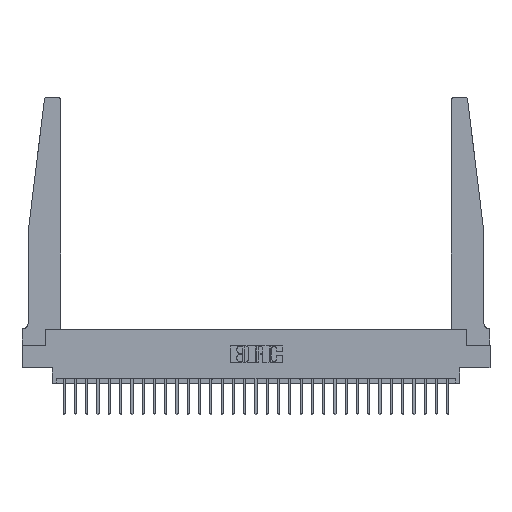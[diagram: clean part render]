
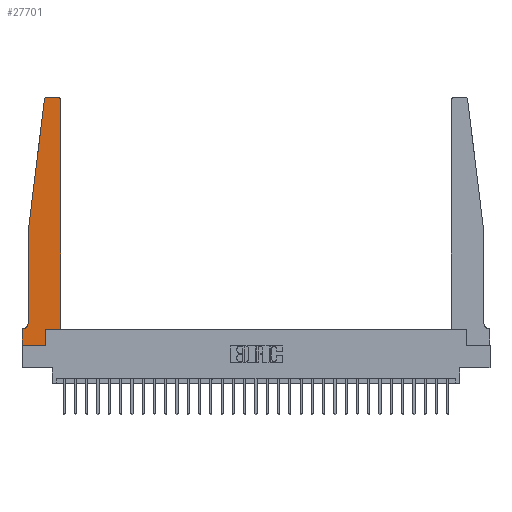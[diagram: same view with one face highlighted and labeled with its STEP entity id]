
A CAD part, top view. The second image highlights one B-rep face of the part: STEP entity #27701.
In plain terms, the highlighted planar face has unit normal (0, 0, 1).
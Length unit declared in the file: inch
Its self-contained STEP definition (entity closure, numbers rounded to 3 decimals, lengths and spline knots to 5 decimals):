
#73 = DIRECTION ( 'NONE',  ( 1., 0., 0. ) ) ;
#163 = EDGE_CURVE ( 'NONE', #21040, #22518, #10459, .T. ) ;
#365 = CARTESIAN_POINT ( 'NONE',  ( 0., 0.1875, 0.37 ) ) ;
#711 = AXIS2_PLACEMENT_3D ( 'NONE', #4234, #19863, #17510 ) ;
#862 = CARTESIAN_POINT ( 'NONE',  ( 0.065, 0.1875, 0.37 ) ) ;
#881 = ORIENTED_EDGE ( 'NONE', *, *, #22320, .T. ) ;
#935 = AXIS2_PLACEMENT_3D ( 'NONE', #18233, #27815, #20877 ) ;
#1850 = CARTESIAN_POINT ( 'NONE',  ( 0.065, 1.25, 0.37 ) ) ;
#1932 = VERTEX_POINT ( 'NONE', #9917 ) ;
#2770 = DIRECTION ( 'NONE',  ( -1., 0., 0. ) ) ;
#3174 = LINE ( 'NONE', #5829, #12867 ) ;
#3251 = VERTEX_POINT ( 'NONE', #11386 ) ;
#3259 = VERTEX_POINT ( 'NONE', #11244 ) ;
#3402 = VERTEX_POINT ( 'NONE', #12240 ) ;
#3509 = DIRECTION ( 'NONE',  ( -0.122, -0.992, 0. ) ) ;
#3838 = VECTOR ( 'NONE', #12747, 39.37008 ) ;
#4233 = CARTESIAN_POINT ( 'NONE',  ( 0.2605, 0., 0.37 ) ) ;
#4234 = CARTESIAN_POINT ( 'NONE',  ( 0.015, 0.2375, 0.37 ) ) ;
#4310 = AXIS2_PLACEMENT_3D ( 'NONE', #365, #22187, #73 ) ;
#5100 = EDGE_LOOP ( 'NONE', ( #24812, #6718, #881, #24952, #23023, #23463, #5910, #11214, #28341, #9028, #5657, #17449 ) ) ;
#5166 = DIRECTION ( 'NONE',  ( -1., 0., 0. ) ) ;
#5617 = EDGE_CURVE ( 'NONE', #22518, #3259, #21421, .T. ) ;
#5657 = ORIENTED_EDGE ( 'NONE', *, *, #10068, .T. ) ;
#5829 = CARTESIAN_POINT ( 'NONE',  ( 0.2605, 0.18, 0.37 ) ) ;
#5910 = ORIENTED_EDGE ( 'NONE', *, *, #23990, .T. ) ;
#5997 = EDGE_CURVE ( 'NONE', #26243, #26681, #3174, .T. ) ;
#6176 = CARTESIAN_POINT ( 'NONE',  ( 0.065, 0.2375, 0.37 ) ) ;
#6427 = DIRECTION ( 'NONE',  ( 1., 0., 0. ) ) ;
#6718 = ORIENTED_EDGE ( 'NONE', *, *, #10291, .T. ) ;
#6726 = VERTEX_POINT ( 'NONE', #6966 ) ;
#6865 = AXIS2_PLACEMENT_3D ( 'NONE', #16122, #15843, #8772 ) ;
#6966 = CARTESIAN_POINT ( 'NONE',  ( 0.395, 2.75, 0.37 ) ) ;
#7486 = EDGE_CURVE ( 'NONE', #3251, #26243, #28417, .T. ) ;
#8772 = DIRECTION ( 'NONE',  ( 1., 0., 0. ) ) ;
#9028 = ORIENTED_EDGE ( 'NONE', *, *, #27541, .T. ) ;
#9371 = VECTOR ( 'NONE', #17293, 39.37008 ) ;
#9666 = VECTOR ( 'NONE', #2770, 39.37008 ) ;
#9760 = VERTEX_POINT ( 'NONE', #28784 ) ;
#9917 = CARTESIAN_POINT ( 'NONE',  ( 0.27653, 2.75, 0.37 ) ) ;
#10068 = EDGE_CURVE ( 'NONE', #10668, #9760, #12353, .T. ) ;
#10291 = EDGE_CURVE ( 'NONE', #1932, #3402, #17422, .T. ) ;
#10459 = LINE ( 'NONE', #28171, #25637 ) ;
#10668 = VERTEX_POINT ( 'NONE', #22879 ) ;
#11214 = ORIENTED_EDGE ( 'NONE', *, *, #7486, .T. ) ;
#11244 = CARTESIAN_POINT ( 'NONE',  ( 0.015, 0.1875, 0.37 ) ) ;
#11386 = CARTESIAN_POINT ( 'NONE',  ( 0., 0., 0.37 ) ) ;
#11794 = CARTESIAN_POINT ( 'NONE',  ( 0.25, 2.75, 0.37 ) ) ;
#12169 = DIRECTION ( 'NONE',  ( 0., 1., 0. ) ) ;
#12218 = LINE ( 'NONE', #14584, #18756 ) ;
#12240 = CARTESIAN_POINT ( 'NONE',  ( 0.24675, 2.72367, 0.37 ) ) ;
#12353 = LINE ( 'NONE', #25790, #18884 ) ;
#12489 = CIRCLE ( 'NONE', #6865, 0.03 ) ;
#12747 = DIRECTION ( 'NONE',  ( 1., 0., 0. ) ) ;
#12867 = VECTOR ( 'NONE', #12169, 39.37008 ) ;
#14584 = CARTESIAN_POINT ( 'NONE',  ( 0.065, 1.25, 0.37 ) ) ;
#15843 = DIRECTION ( 'NONE',  ( 0., 0., 1. ) ) ;
#16122 = CARTESIAN_POINT ( 'NONE',  ( 0.395, 2.72, 0.37 ) ) ;
#16228 = LINE ( 'NONE', #11794, #22544 ) ;
#16712 = LINE ( 'NONE', #23620, #9371 ) ;
#17106 = EDGE_CURVE ( 'NONE', #9760, #6726, #12489, .T. ) ;
#17293 = DIRECTION ( 'NONE',  ( 0., -1., 0. ) ) ;
#17422 = CIRCLE ( 'NONE', #935, 0.03 ) ;
#17449 = ORIENTED_EDGE ( 'NONE', *, *, #17106, .T. ) ;
#17510 = DIRECTION ( 'NONE',  ( -1., 0., 0. ) ) ;
#17772 = CARTESIAN_POINT ( 'NONE',  ( 0., 0., 0.37 ) ) ;
#18233 = CARTESIAN_POINT ( 'NONE',  ( 0.27653, 2.72, 0.37 ) ) ;
#18700 = LINE ( 'NONE', #862, #9666 ) ;
#18756 = VECTOR ( 'NONE', #3509, 39.37008 ) ;
#18884 = VECTOR ( 'NONE', #19576, 39.37008 ) ;
#18886 = EDGE_CURVE ( 'NONE', #3259, #24795, #18700, .T. ) ;
#19576 = DIRECTION ( 'NONE',  ( 0., 1., 0. ) ) ;
#19863 = DIRECTION ( 'NONE',  ( 0., 0., -1. ) ) ;
#19985 = PLANE ( 'NONE',  #4310 ) ;
#20385 = VECTOR ( 'NONE', #6427, 39.37008 ) ;
#20877 = DIRECTION ( 'NONE',  ( 1., 0., 0. ) ) ;
#21040 = VERTEX_POINT ( 'NONE', #1850 ) ;
#21370 = DIRECTION ( 'NONE',  ( 0., -1., 0. ) ) ;
#21421 = CIRCLE ( 'NONE', #711, 0.05 ) ;
#22187 = DIRECTION ( 'NONE',  ( 0., 0., 1. ) ) ;
#22320 = EDGE_CURVE ( 'NONE', #3402, #21040, #12218, .T. ) ;
#22518 = VERTEX_POINT ( 'NONE', #6176 ) ;
#22544 = VECTOR ( 'NONE', #5166, 39.37008 ) ;
#22879 = CARTESIAN_POINT ( 'NONE',  ( 0.425, 0.18, 0.37 ) ) ;
#23006 = EDGE_CURVE ( 'NONE', #6726, #1932, #16228, .T. ) ;
#23023 = ORIENTED_EDGE ( 'NONE', *, *, #5617, .T. ) ;
#23463 = ORIENTED_EDGE ( 'NONE', *, *, #18886, .T. ) ;
#23620 = CARTESIAN_POINT ( 'NONE',  ( 0., 0., 0.37 ) ) ;
#23990 = EDGE_CURVE ( 'NONE', #24795, #3251, #16712, .T. ) ;
#24266 = LINE ( 'NONE', #28401, #3838 ) ;
#24795 = VERTEX_POINT ( 'NONE', #25198 ) ;
#24812 = ORIENTED_EDGE ( 'NONE', *, *, #23006, .T. ) ;
#24952 = ORIENTED_EDGE ( 'NONE', *, *, #163, .T. ) ;
#25198 = CARTESIAN_POINT ( 'NONE',  ( 0., 0.1875, 0.37 ) ) ;
#25637 = VECTOR ( 'NONE', #21370, 39.37008 ) ;
#25790 = CARTESIAN_POINT ( 'NONE',  ( 0.425, 0.18, 0.37 ) ) ;
#26243 = VERTEX_POINT ( 'NONE', #4233 ) ;
#26681 = VERTEX_POINT ( 'NONE', #27478 ) ;
#26927 = FACE_OUTER_BOUND ( 'NONE', #5100, .T. ) ;
#27478 = CARTESIAN_POINT ( 'NONE',  ( 0.2605, 0.18, 0.37 ) ) ;
#27541 = EDGE_CURVE ( 'NONE', #26681, #10668, #24266, .T. ) ;
#27701 = ADVANCED_FACE ( 'NONE', ( #26927 ), #19985, .T. ) ;
#27815 = DIRECTION ( 'NONE',  ( 0., 0., 1. ) ) ;
#28171 = CARTESIAN_POINT ( 'NONE',  ( 0.065, 1.25, 0.37 ) ) ;
#28341 = ORIENTED_EDGE ( 'NONE', *, *, #5997, .T. ) ;
#28401 = CARTESIAN_POINT ( 'NONE',  ( 0.425, 0.18, 0.37 ) ) ;
#28417 = LINE ( 'NONE', #17772, #20385 ) ;
#28784 = CARTESIAN_POINT ( 'NONE',  ( 0.425, 2.72, 0.37 ) ) ;
